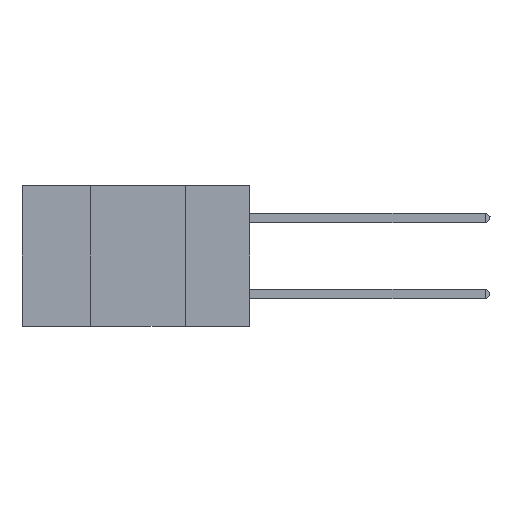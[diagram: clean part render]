
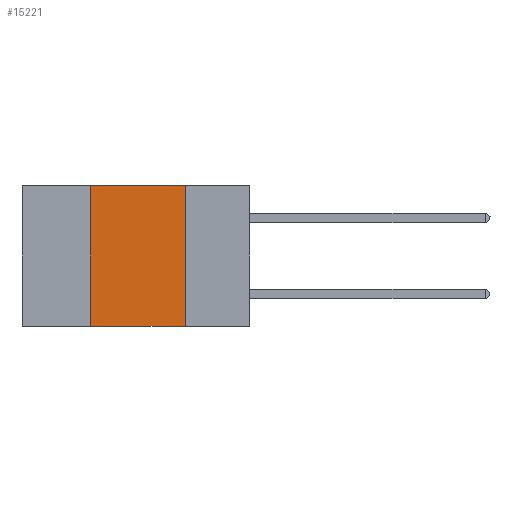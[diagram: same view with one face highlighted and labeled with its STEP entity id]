
A CAD part, left-side view. The second image highlights one B-rep face of the part: STEP entity #15221.
In plain terms, the highlighted planar face has unit normal (-1, 0, 0).
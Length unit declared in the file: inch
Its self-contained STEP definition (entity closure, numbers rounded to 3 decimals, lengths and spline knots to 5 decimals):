
#97 = VERTEX_POINT ( 'NONE', #5162 ) ;
#648 = DIRECTION ( 'NONE',  ( 0., 0., -1. ) ) ;
#688 = CARTESIAN_POINT ( 'NONE',  ( 0., 0.6, 0. ) ) ;
#1618 = VERTEX_POINT ( 'NONE', #4145 ) ;
#2537 = DIRECTION ( 'NONE',  ( 0., -1., 0. ) ) ;
#3066 = ORIENTED_EDGE ( 'NONE', *, *, #5772, .F. ) ;
#3284 = ORIENTED_EDGE ( 'NONE', *, *, #10859, .F. ) ;
#4145 = CARTESIAN_POINT ( 'NONE',  ( 0., 0.17, 0. ) ) ;
#4176 = VECTOR ( 'NONE', #648, 39.37008 ) ;
#4627 = CARTESIAN_POINT ( 'NONE',  ( 0., 0.42, -0.37 ) ) ;
#4891 = DIRECTION ( 'NONE',  ( 0., 0., -1. ) ) ;
#4969 = CARTESIAN_POINT ( 'NONE',  ( 0., 0.6, 0. ) ) ;
#5162 = CARTESIAN_POINT ( 'NONE',  ( 0., 0.17, -0.37 ) ) ;
#5617 = DIRECTION ( 'NONE',  ( 0., -1., 0. ) ) ;
#5772 = EDGE_CURVE ( 'NONE', #11669, #15094, #11006, .T. ) ;
#6170 = LINE ( 'NONE', #13645, #10719 ) ;
#6787 = LINE ( 'NONE', #11739, #4176 ) ;
#7322 = FACE_OUTER_BOUND ( 'NONE', #10710, .T. ) ;
#8117 = AXIS2_PLACEMENT_3D ( 'NONE', #4969, #9739, #4891 ) ;
#8344 = ORIENTED_EDGE ( 'NONE', *, *, #9997, .F. ) ;
#8650 = CARTESIAN_POINT ( 'NONE',  ( 0., 0.42, 0. ) ) ;
#9739 = DIRECTION ( 'NONE',  ( 1., 0., 0. ) ) ;
#9997 = EDGE_CURVE ( 'NONE', #15094, #1618, #11786, .T. ) ;
#10710 = EDGE_LOOP ( 'NONE', ( #3284, #8344, #3066, #11859 ) ) ;
#10719 = VECTOR ( 'NONE', #2537, 39.37008 ) ;
#10723 = CARTESIAN_POINT ( 'NONE',  ( 0., 0.42, 0. ) ) ;
#10859 = EDGE_CURVE ( 'NONE', #1618, #97, #6787, .T. ) ;
#11006 = LINE ( 'NONE', #8650, #12805 ) ;
#11669 = VERTEX_POINT ( 'NONE', #4627 ) ;
#11739 = CARTESIAN_POINT ( 'NONE',  ( 0., 0.17, 0. ) ) ;
#11786 = LINE ( 'NONE', #688, #14827 ) ;
#11859 = ORIENTED_EDGE ( 'NONE', *, *, #13944, .T. ) ;
#12273 = PLANE ( 'NONE',  #8117 ) ;
#12805 = VECTOR ( 'NONE', #15946, 39.37008 ) ;
#13645 = CARTESIAN_POINT ( 'NONE',  ( 0., 0.6, -0.37 ) ) ;
#13944 = EDGE_CURVE ( 'NONE', #11669, #97, #6170, .T. ) ;
#14827 = VECTOR ( 'NONE', #5617, 39.37008 ) ;
#15094 = VERTEX_POINT ( 'NONE', #10723 ) ;
#15221 = ADVANCED_FACE ( 'NONE', ( #7322 ), #12273, .F. ) ;
#15946 = DIRECTION ( 'NONE',  ( 0., 0., 1. ) ) ;
